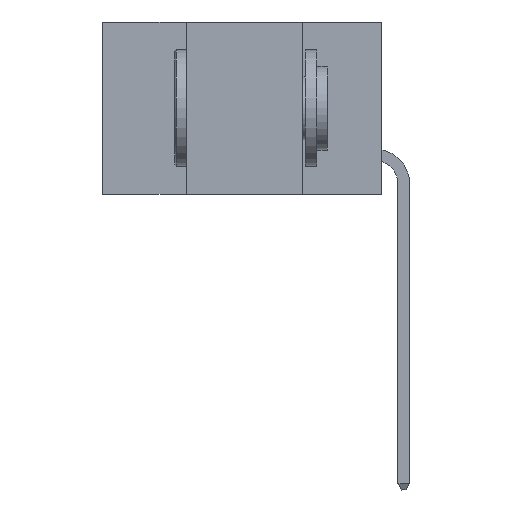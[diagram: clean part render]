
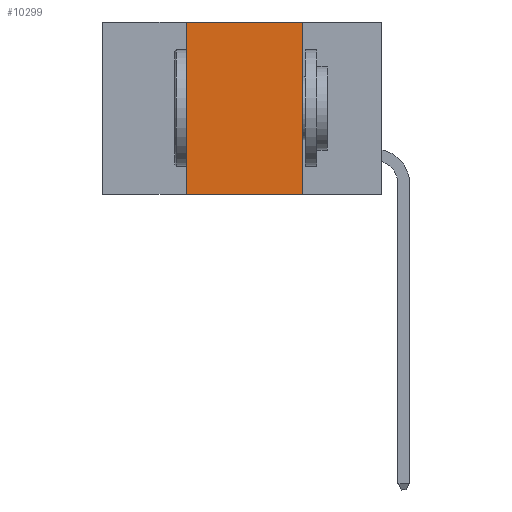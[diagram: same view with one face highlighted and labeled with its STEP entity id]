
A CAD part, left-side view. The second image highlights one B-rep face of the part: STEP entity #10299.
In plain terms, the highlighted planar face has unit normal (-1, 0, 0).
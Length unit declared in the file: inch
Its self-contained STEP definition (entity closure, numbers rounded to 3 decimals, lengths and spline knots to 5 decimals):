
#32 = VECTOR ( 'NONE', #10519, 39.37008 ) ;
#588 = DIRECTION ( 'NONE',  ( 0., -1., 0. ) ) ;
#663 = VECTOR ( 'NONE', #2722, 39.37008 ) ;
#961 = LINE ( 'NONE', #8312, #663 ) ;
#984 = AXIS2_PLACEMENT_3D ( 'NONE', #9487, #7687, #2012 ) ;
#1706 = EDGE_CURVE ( 'NONE', #3007, #6640, #5257, .T. ) ;
#2012 = DIRECTION ( 'NONE',  ( 0., 0., -1. ) ) ;
#2287 = ORIENTED_EDGE ( 'NONE', *, *, #6971, .F. ) ;
#2722 = DIRECTION ( 'NONE',  ( 0., 0., 1. ) ) ;
#3007 = VERTEX_POINT ( 'NONE', #9452 ) ;
#3188 = CARTESIAN_POINT ( 'NONE',  ( 0., 0.17, 0. ) ) ;
#3363 = EDGE_CURVE ( 'NONE', #11786, #6640, #12042, .T. ) ;
#3704 = LINE ( 'NONE', #11716, #10755 ) ;
#3728 = CARTESIAN_POINT ( 'NONE',  ( 0., 0.17, 0. ) ) ;
#3856 = DIRECTION ( 'NONE',  ( 0., 0., -1. ) ) ;
#4527 = ORIENTED_EDGE ( 'NONE', *, *, #8670, .F. ) ;
#5126 = CARTESIAN_POINT ( 'NONE',  ( 0., 0.17, -0.37 ) ) ;
#5257 = LINE ( 'NONE', #9671, #32 ) ;
#6640 = VERTEX_POINT ( 'NONE', #5126 ) ;
#6714 = ORIENTED_EDGE ( 'NONE', *, *, #3363, .F. ) ;
#6971 = EDGE_CURVE ( 'NONE', #3007, #8720, #961, .T. ) ;
#7320 = ORIENTED_EDGE ( 'NONE', *, *, #1706, .T. ) ;
#7636 = VECTOR ( 'NONE', #3856, 39.37008 ) ;
#7651 = PLANE ( 'NONE',  #984 ) ;
#7687 = DIRECTION ( 'NONE',  ( 1., 0., 0. ) ) ;
#8312 = CARTESIAN_POINT ( 'NONE',  ( 0., 0.42, 0. ) ) ;
#8670 = EDGE_CURVE ( 'NONE', #8720, #11786, #3704, .T. ) ;
#8720 = VERTEX_POINT ( 'NONE', #9718 ) ;
#9452 = CARTESIAN_POINT ( 'NONE',  ( 0., 0.42, -0.37 ) ) ;
#9487 = CARTESIAN_POINT ( 'NONE',  ( 0., 0.6, 0. ) ) ;
#9496 = FACE_OUTER_BOUND ( 'NONE', #10964, .T. ) ;
#9671 = CARTESIAN_POINT ( 'NONE',  ( 0., 0.6, -0.37 ) ) ;
#9718 = CARTESIAN_POINT ( 'NONE',  ( 0., 0.42, 0. ) ) ;
#10299 = ADVANCED_FACE ( 'NONE', ( #9496 ), #7651, .F. ) ;
#10519 = DIRECTION ( 'NONE',  ( 0., -1., 0. ) ) ;
#10755 = VECTOR ( 'NONE', #588, 39.37008 ) ;
#10964 = EDGE_LOOP ( 'NONE', ( #6714, #4527, #2287, #7320 ) ) ;
#11716 = CARTESIAN_POINT ( 'NONE',  ( 0., 0.6, 0. ) ) ;
#11786 = VERTEX_POINT ( 'NONE', #3188 ) ;
#12042 = LINE ( 'NONE', #3728, #7636 ) ;
